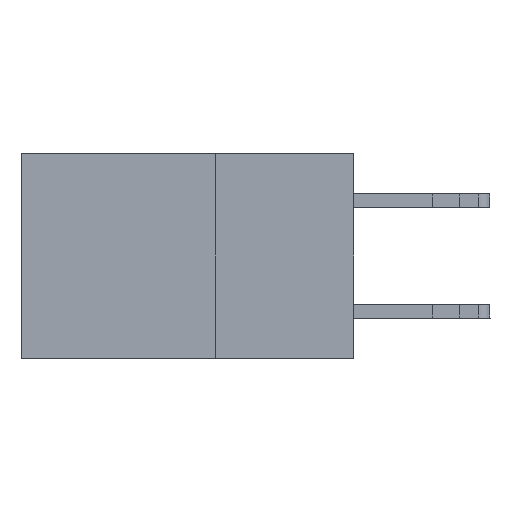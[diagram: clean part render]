
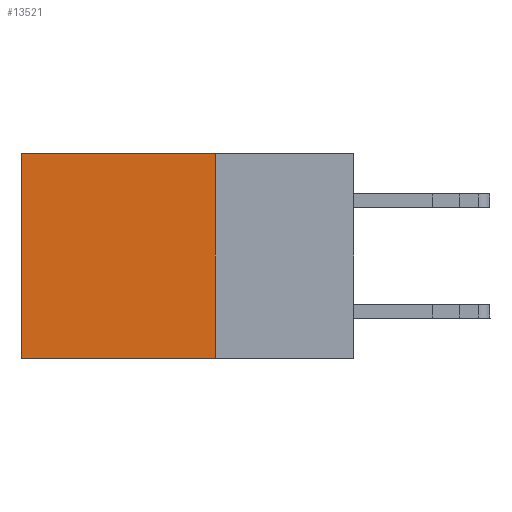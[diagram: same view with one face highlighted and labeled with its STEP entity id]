
A CAD part, left-side view. The second image highlights one B-rep face of the part: STEP entity #13521.
In plain terms, the highlighted planar face has unit normal (-1, 0, 0).
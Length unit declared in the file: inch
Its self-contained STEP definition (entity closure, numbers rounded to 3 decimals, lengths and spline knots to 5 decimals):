
#460 = EDGE_CURVE ( 'NONE', #23140, #1410, #1815, .T. ) ;
#1347 = DIRECTION ( 'NONE',  ( 0., 0., -1. ) ) ;
#1410 = VERTEX_POINT ( 'NONE', #24627 ) ;
#1815 = LINE ( 'NONE', #6555, #4175 ) ;
#2017 = DIRECTION ( 'NONE',  ( 1., 0., 0. ) ) ;
#2223 = ORIENTED_EDGE ( 'NONE', *, *, #460, .T. ) ;
#4175 = VECTOR ( 'NONE', #22476, 39.37008 ) ;
#4810 = VECTOR ( 'NONE', #1347, 39.37008 ) ;
#5780 = VECTOR ( 'NONE', #16051, 39.37008 ) ;
#6457 = EDGE_LOOP ( 'NONE', ( #17213, #25968, #20770, #2223 ) ) ;
#6555 = CARTESIAN_POINT ( 'NONE',  ( 0.2875, 0.25, 0. ) ) ;
#6762 = CARTESIAN_POINT ( 'NONE',  ( 0.2875, 0.25, 0. ) ) ;
#8112 = DIRECTION ( 'NONE',  ( 0., 1., 0. ) ) ;
#8242 = LINE ( 'NONE', #14613, #12067 ) ;
#9946 = LINE ( 'NONE', #18033, #5780 ) ;
#11221 = AXIS2_PLACEMENT_3D ( 'NONE', #24297, #2017, #22306 ) ;
#11911 = CARTESIAN_POINT ( 'NONE',  ( 0.2875, 0.25, -0.37 ) ) ;
#12067 = VECTOR ( 'NONE', #8112, 39.37008 ) ;
#13021 = EDGE_CURVE ( 'NONE', #17505, #22028, #8242, .T. ) ;
#13521 = ADVANCED_FACE ( 'NONE', ( #20061 ), #24416, .F. ) ;
#14613 = CARTESIAN_POINT ( 'NONE',  ( 0.2875, 0.25, -0.37 ) ) ;
#16051 = DIRECTION ( 'NONE',  ( 0., 0., -1. ) ) ;
#16986 = EDGE_CURVE ( 'NONE', #1410, #22028, #21511, .T. ) ;
#17213 = ORIENTED_EDGE ( 'NONE', *, *, #16986, .T. ) ;
#17505 = VERTEX_POINT ( 'NONE', #11911 ) ;
#18033 = CARTESIAN_POINT ( 'NONE',  ( 0.2875, 0.25, 0. ) ) ;
#20061 = FACE_OUTER_BOUND ( 'NONE', #6457, .T. ) ;
#20331 = EDGE_CURVE ( 'NONE', #23140, #17505, #9946, .T. ) ;
#20770 = ORIENTED_EDGE ( 'NONE', *, *, #20331, .F. ) ;
#21511 = LINE ( 'NONE', #21641, #4810 ) ;
#21641 = CARTESIAN_POINT ( 'NONE',  ( 0.2875, 0.6, 0. ) ) ;
#22028 = VERTEX_POINT ( 'NONE', #25979 ) ;
#22306 = DIRECTION ( 'NONE',  ( 0., 0., -1. ) ) ;
#22476 = DIRECTION ( 'NONE',  ( 0., 1., 0. ) ) ;
#23140 = VERTEX_POINT ( 'NONE', #6762 ) ;
#24297 = CARTESIAN_POINT ( 'NONE',  ( 0.2875, 0.25, 0. ) ) ;
#24416 = PLANE ( 'NONE',  #11221 ) ;
#24627 = CARTESIAN_POINT ( 'NONE',  ( 0.2875, 0.6, 0. ) ) ;
#25968 = ORIENTED_EDGE ( 'NONE', *, *, #13021, .F. ) ;
#25979 = CARTESIAN_POINT ( 'NONE',  ( 0.2875, 0.6, -0.37 ) ) ;
